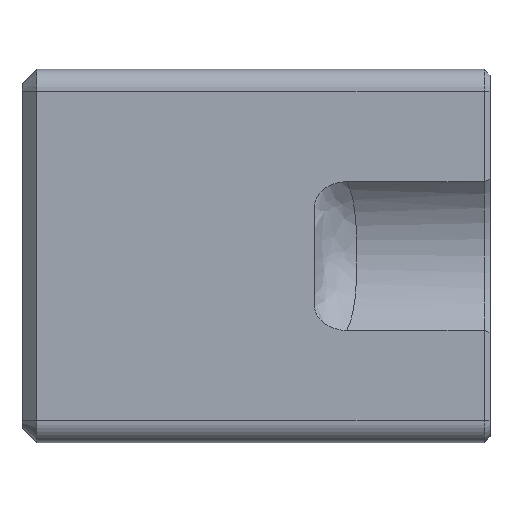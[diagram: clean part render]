
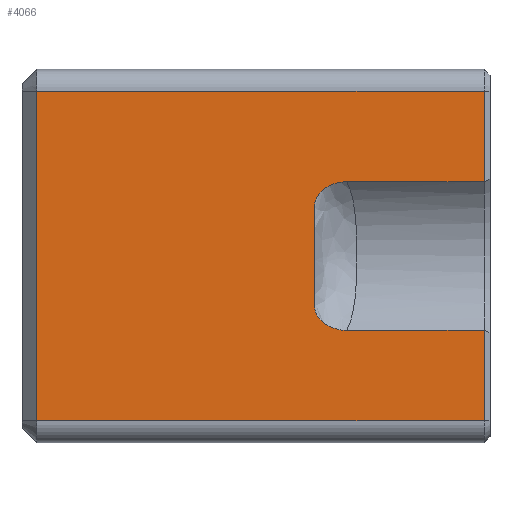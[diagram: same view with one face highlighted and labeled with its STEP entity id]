
A CAD part, front view. The second image highlights one B-rep face of the part: STEP entity #4066.
In plain terms, the highlighted planar face has unit normal (0, -1, 0).
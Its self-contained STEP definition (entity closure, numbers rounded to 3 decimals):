
#529=B_SPLINE_CURVE_WITH_KNOTS('',3,(#11583,#11584,#11585,#11586,#11587,
#11588,#11589,#11590,#11591,#11592,#11593,#11594,#11595,#11596,#11597,#11598,
#11599,#11600,#11601,#11602),.UNSPECIFIED.,.F.,.F.,(4,2,2,2,2,2,2,2,2,4),
(0.,0.,0.,0.002,0.006,
0.014,0.03,0.065,0.119,
0.177),.UNSPECIFIED.);
#530=B_SPLINE_CURVE_WITH_KNOTS('',3,(#11606,#11607,#11608,#11609,#11610,
#11611,#11612,#11613,#11614,#11615,#11616,#11617,#11618,#11619,#11620,#11621,
#11622,#11623,#11624,#11625),.UNSPECIFIED.,.F.,.F.,(4,2,2,2,2,2,2,2,2,4),
(0.,0.102,0.197,0.257,0.286,
0.3,0.306,0.31,0.31,
0.31),.UNSPECIFIED.);
#583=PLANE('',#4347);
#880=FACE_OUTER_BOUND('',#1127,.T.);
#1127=EDGE_LOOP('',(#3737,#3738,#3739,#3740,#3741,#3742,#3743,#3744,#3745,
#3746));
#1233=LINE('',#11550,#1350);
#1242=LINE('',#11572,#1359);
#1243=LINE('',#11577,#1360);
#1244=LINE('',#11581,#1361);
#1245=LINE('',#11604,#1362);
#1246=LINE('',#11626,#1363);
#1247=LINE('',#11628,#1364);
#1248=LINE('',#11629,#1365);
#1350=VECTOR('',#4905,10.);
#1359=VECTOR('',#4938,10.);
#1360=VECTOR('',#4945,10.);
#1361=VECTOR('',#4950,10.);
#1362=VECTOR('',#4951,10.);
#1363=VECTOR('',#4952,10.);
#1364=VECTOR('',#4953,10.);
#1365=VECTOR('',#4954,10.);
#1894=VERTEX_POINT('',#11537);
#1895=VERTEX_POINT('',#11542);
#1896=VERTEX_POINT('',#11549);
#1897=VERTEX_POINT('',#11568);
#1898=VERTEX_POINT('',#11576);
#1899=VERTEX_POINT('',#11580);
#1900=VERTEX_POINT('',#11582);
#1901=VERTEX_POINT('',#11603);
#1902=VERTEX_POINT('',#11605);
#1903=VERTEX_POINT('',#11627);
#2502=EDGE_CURVE('',#1895,#1896,#1233,.T.);
#2515=EDGE_CURVE('',#1897,#1894,#1242,.T.);
#2517=EDGE_CURVE('',#1896,#1898,#1243,.T.);
#2519=EDGE_CURVE('',#1895,#1899,#1244,.T.);
#2520=EDGE_CURVE('',#1900,#1899,#529,.T.);
#2521=EDGE_CURVE('',#1900,#1901,#1245,.T.);
#2522=EDGE_CURVE('',#1901,#1902,#530,.F.);
#2523=EDGE_CURVE('',#1902,#1894,#1246,.T.);
#2524=EDGE_CURVE('',#1903,#1897,#1247,.T.);
#2525=EDGE_CURVE('',#1898,#1903,#1248,.T.);
#3737=ORIENTED_EDGE('',*,*,#2502,.F.);
#3738=ORIENTED_EDGE('',*,*,#2519,.T.);
#3739=ORIENTED_EDGE('',*,*,#2520,.F.);
#3740=ORIENTED_EDGE('',*,*,#2521,.T.);
#3741=ORIENTED_EDGE('',*,*,#2522,.T.);
#3742=ORIENTED_EDGE('',*,*,#2523,.T.);
#3743=ORIENTED_EDGE('',*,*,#2515,.F.);
#3744=ORIENTED_EDGE('',*,*,#2524,.F.);
#3745=ORIENTED_EDGE('',*,*,#2525,.F.);
#3746=ORIENTED_EDGE('',*,*,#2517,.F.);
#4066=ADVANCED_FACE('',(#880),#583,.T.);
#4347=AXIS2_PLACEMENT_3D('',#11579,#4948,#4949);
#4905=DIRECTION('',(0.,0.,-1.));
#4938=DIRECTION('',(0.,0.,-1.));
#4945=DIRECTION('',(-1.,0.,0.));
#4948=DIRECTION('center_axis',(0.,-1.,0.));
#4949=DIRECTION('ref_axis',(0.,0.,1.));
#4950=DIRECTION('',(-1.,0.,0.));
#4951=DIRECTION('',(0.,0.,1.));
#4952=DIRECTION('',(1.,0.,0.));
#4953=DIRECTION('',(1.,0.,0.));
#4954=DIRECTION('',(0.,0.,1.));
#11537=CARTESIAN_POINT('',(-183.534,-11.455,5.083));
#11542=CARTESIAN_POINT('',(-183.534,-11.455,-5.083));
#11549=CARTESIAN_POINT('',(-183.534,-11.455,-11.264));
#11550=CARTESIAN_POINT('',(-183.534,-11.455,-6.128));
#11568=CARTESIAN_POINT('',(-183.534,-11.455,11.264));
#11572=CARTESIAN_POINT('',(-183.534,-11.455,-6.128));
#11576=CARTESIAN_POINT('',(-214.134,-11.455,-11.264));
#11577=CARTESIAN_POINT('',(-183.134,-11.455,-11.264));
#11579=CARTESIAN_POINT('Origin',(-183.134,-11.455,-12.256));
#11580=CARTESIAN_POINT('',(-192.94,-11.455,-5.083));
#11581=CARTESIAN_POINT('',(-183.134,-11.455,-5.083));
#11582=CARTESIAN_POINT('',(-195.134,-11.455,-3.546));
#11583=CARTESIAN_POINT('Ctrl Pts',(-195.134,-11.455,-3.546));
#11584=CARTESIAN_POINT('Ctrl Pts',(-195.134,-11.455,-3.546));
#11585=CARTESIAN_POINT('Ctrl Pts',(-195.134,-11.455,-3.547));
#11586=CARTESIAN_POINT('Ctrl Pts',(-195.134,-11.455,-3.548));
#11587=CARTESIAN_POINT('Ctrl Pts',(-195.134,-11.455,-3.549));
#11588=CARTESIAN_POINT('Ctrl Pts',(-195.134,-11.455,-3.557));
#11589=CARTESIAN_POINT('Ctrl Pts',(-195.133,-11.455,-3.565));
#11590=CARTESIAN_POINT('Ctrl Pts',(-195.13,-11.455,-3.592));
#11591=CARTESIAN_POINT('Ctrl Pts',(-195.127,-11.455,-3.61));
#11592=CARTESIAN_POINT('Ctrl Pts',(-195.116,-11.455,-3.667));
#11593=CARTESIAN_POINT('Ctrl Pts',(-195.105,-11.455,-3.707));
#11594=CARTESIAN_POINT('Ctrl Pts',(-195.066,-11.455,-3.826));
#11595=CARTESIAN_POINT('Ctrl Pts',(-195.031,-11.455,-3.905));
#11596=CARTESIAN_POINT('Ctrl Pts',(-194.907,-11.455,-4.136));
#11597=CARTESIAN_POINT('Ctrl Pts',(-194.797,-11.455,-4.279));
#11598=CARTESIAN_POINT('Ctrl Pts',(-194.473,-11.455,
-4.603));
#11599=CARTESIAN_POINT('Ctrl Pts',(-194.224,-11.455,-4.771));
#11600=CARTESIAN_POINT('Ctrl Pts',(-193.619,-11.455,-5.02));
#11601=CARTESIAN_POINT('Ctrl Pts',(-193.281,-11.455,-5.083));
#11602=CARTESIAN_POINT('Ctrl Pts',(-192.94,-11.455,-5.083));
#11603=CARTESIAN_POINT('',(-195.134,-11.455,3.546));
#11604=CARTESIAN_POINT('',(-195.134,-11.455,-6.128));
#11605=CARTESIAN_POINT('',(-192.94,-11.455,5.083));
#11606=CARTESIAN_POINT('Ctrl Pts',(-192.94,-11.455,5.083));
#11607=CARTESIAN_POINT('Ctrl Pts',(-193.281,-11.455,5.083));
#11608=CARTESIAN_POINT('Ctrl Pts',(-193.619,-11.455,5.02));
#11609=CARTESIAN_POINT('Ctrl Pts',(-194.224,-11.455,4.771));
#11610=CARTESIAN_POINT('Ctrl Pts',(-194.473,-11.455,4.603));
#11611=CARTESIAN_POINT('Ctrl Pts',(-194.797,-11.455,4.279));
#11612=CARTESIAN_POINT('Ctrl Pts',(-194.907,-11.455,4.136));
#11613=CARTESIAN_POINT('Ctrl Pts',(-195.031,-11.455,3.905));
#11614=CARTESIAN_POINT('Ctrl Pts',(-195.066,-11.455,3.826));
#11615=CARTESIAN_POINT('Ctrl Pts',(-195.105,-11.455,3.707));
#11616=CARTESIAN_POINT('Ctrl Pts',(-195.116,-11.455,3.667));
#11617=CARTESIAN_POINT('Ctrl Pts',(-195.127,-11.455,3.61));
#11618=CARTESIAN_POINT('Ctrl Pts',(-195.13,-11.455,3.592));
#11619=CARTESIAN_POINT('Ctrl Pts',(-195.133,-11.455,3.565));
#11620=CARTESIAN_POINT('Ctrl Pts',(-195.134,-11.455,3.557));
#11621=CARTESIAN_POINT('Ctrl Pts',(-195.134,-11.455,3.549));
#11622=CARTESIAN_POINT('Ctrl Pts',(-195.134,-11.455,3.548));
#11623=CARTESIAN_POINT('Ctrl Pts',(-195.134,-11.455,3.547));
#11624=CARTESIAN_POINT('Ctrl Pts',(-195.134,-11.455,3.546));
#11625=CARTESIAN_POINT('Ctrl Pts',(-195.134,-11.455,3.546));
#11626=CARTESIAN_POINT('',(-183.134,-11.455,5.083));
#11627=CARTESIAN_POINT('',(-214.134,-11.455,11.264));
#11628=CARTESIAN_POINT('',(-183.134,-11.455,11.264));
#11629=CARTESIAN_POINT('',(-214.134,-11.455,-6.128));
